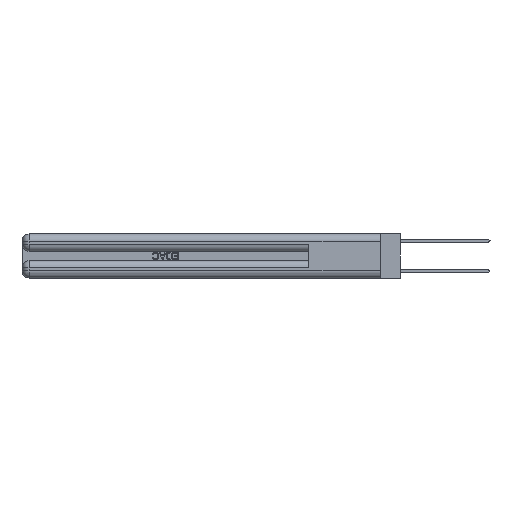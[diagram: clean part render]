
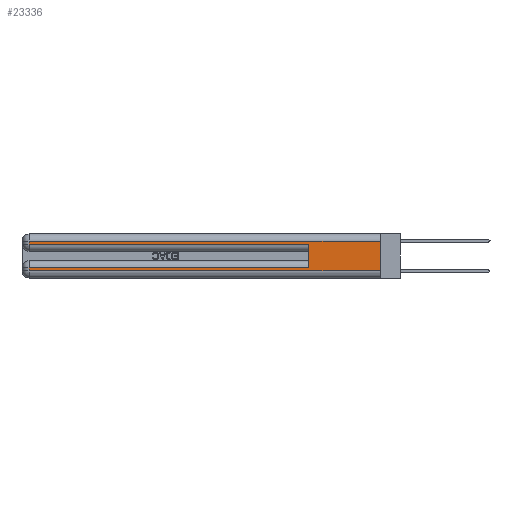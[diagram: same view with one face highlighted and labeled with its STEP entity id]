
A CAD part, left-side view. The second image highlights one B-rep face of the part: STEP entity #23336.
In plain terms, the highlighted planar face has unit normal (-1, 0, 0).
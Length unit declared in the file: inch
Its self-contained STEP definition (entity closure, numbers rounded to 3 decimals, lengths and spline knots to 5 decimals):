
#729 = EDGE_CURVE ( 'NONE', #27378, #1711, #8715, .T. ) ;
#1304 = VECTOR ( 'NONE', #10095, 39.37008 ) ;
#1372 = CARTESIAN_POINT ( 'NONE',  ( 0., 2.94, 0.285 ) ) ;
#1680 = LINE ( 'NONE', #24981, #14937 ) ;
#1711 = VERTEX_POINT ( 'NONE', #3402 ) ;
#1877 = DIRECTION ( 'NONE',  ( 0., 0., 1. ) ) ;
#3402 = CARTESIAN_POINT ( 'NONE',  ( 0., 2.94, 0.06 ) ) ;
#3909 = VECTOR ( 'NONE', #31940, 39.37008 ) ;
#4129 = EDGE_LOOP ( 'NONE', ( #23627, #28329, #7637, #20139, #12692, #15837, #10748, #32167 ) ) ;
#4683 = LINE ( 'NONE', #7664, #8990 ) ;
#4690 = LINE ( 'NONE', #29480, #3909 ) ;
#5422 = CARTESIAN_POINT ( 'NONE',  ( 0., 0., 0.37 ) ) ;
#5751 = VECTOR ( 'NONE', #10068, 39.37008 ) ;
#7191 = VERTEX_POINT ( 'NONE', #12171 ) ;
#7320 = LINE ( 'NONE', #5422, #12373 ) ;
#7637 = ORIENTED_EDGE ( 'NONE', *, *, #17892, .T. ) ;
#7664 = CARTESIAN_POINT ( 'NONE',  ( 0., 0., 0.06 ) ) ;
#7737 = EDGE_CURVE ( 'NONE', #7191, #26913, #4690, .T. ) ;
#8115 = LINE ( 'NONE', #17492, #5751 ) ;
#8715 = LINE ( 'NONE', #27445, #1304 ) ;
#8990 = VECTOR ( 'NONE', #27620, 39.37008 ) ;
#9276 = DIRECTION ( 'NONE',  ( 0., 0., -1. ) ) ;
#9380 = CARTESIAN_POINT ( 'NONE',  ( 0., 0.6, 0.145 ) ) ;
#10068 = DIRECTION ( 'NONE',  ( 0., 1., 0. ) ) ;
#10095 = DIRECTION ( 'NONE',  ( 0., 0., -1. ) ) ;
#10542 = DIRECTION ( 'NONE',  ( 0., 0., -1. ) ) ;
#10748 = ORIENTED_EDGE ( 'NONE', *, *, #729, .T. ) ;
#11470 = VECTOR ( 'NONE', #1877, 39.37008 ) ;
#12171 = CARTESIAN_POINT ( 'NONE',  ( 0., 0., 0.31 ) ) ;
#12373 = VECTOR ( 'NONE', #10542, 39.37008 ) ;
#12692 = ORIENTED_EDGE ( 'NONE', *, *, #30060, .F. ) ;
#13063 = DIRECTION ( 'NONE',  ( 1., 0., 0. ) ) ;
#14129 = FACE_OUTER_BOUND ( 'NONE', #4129, .T. ) ;
#14238 = CARTESIAN_POINT ( 'NONE',  ( 0., 2.94, 0.085 ) ) ;
#14470 = CARTESIAN_POINT ( 'NONE',  ( 0., 0., 0.06 ) ) ;
#14937 = VECTOR ( 'NONE', #27485, 39.37008 ) ;
#15837 = ORIENTED_EDGE ( 'NONE', *, *, #25826, .T. ) ;
#16109 = EDGE_CURVE ( 'NONE', #30717, #17223, #1680, .T. ) ;
#16382 = VECTOR ( 'NONE', #9276, 39.37008 ) ;
#17223 = VERTEX_POINT ( 'NONE', #26765 ) ;
#17453 = EDGE_CURVE ( 'NONE', #1711, #23746, #4683, .T. ) ;
#17492 = CARTESIAN_POINT ( 'NONE',  ( 0., 0., 0.085 ) ) ;
#17892 = EDGE_CURVE ( 'NONE', #26913, #30717, #22989, .T. ) ;
#18104 = LINE ( 'NONE', #9380, #11470 ) ;
#18151 = AXIS2_PLACEMENT_3D ( 'NONE', #28008, #13063, #30479 ) ;
#18774 = CARTESIAN_POINT ( 'NONE',  ( 0., 0.6, 0.085 ) ) ;
#19071 = CARTESIAN_POINT ( 'NONE',  ( 0., 2.94, 0.31 ) ) ;
#19201 = CARTESIAN_POINT ( 'NONE',  ( 0., 2.94, 0.37 ) ) ;
#20139 = ORIENTED_EDGE ( 'NONE', *, *, #16109, .T. ) ;
#22971 = PLANE ( 'NONE',  #18151 ) ;
#22989 = LINE ( 'NONE', #19201, #16382 ) ;
#23336 = ADVANCED_FACE ( 'NONE', ( #14129 ), #22971, .F. ) ;
#23627 = ORIENTED_EDGE ( 'NONE', *, *, #28419, .F. ) ;
#23746 = VERTEX_POINT ( 'NONE', #14470 ) ;
#24981 = CARTESIAN_POINT ( 'NONE',  ( 0., 0., 0.285 ) ) ;
#25826 = EDGE_CURVE ( 'NONE', #27901, #27378, #8115, .T. ) ;
#26765 = CARTESIAN_POINT ( 'NONE',  ( 0., 0.6, 0.285 ) ) ;
#26913 = VERTEX_POINT ( 'NONE', #19071 ) ;
#27378 = VERTEX_POINT ( 'NONE', #14238 ) ;
#27445 = CARTESIAN_POINT ( 'NONE',  ( 0., 2.94, 0.37 ) ) ;
#27485 = DIRECTION ( 'NONE',  ( 0., -1., 0. ) ) ;
#27620 = DIRECTION ( 'NONE',  ( 0., -1., 0. ) ) ;
#27901 = VERTEX_POINT ( 'NONE', #18774 ) ;
#28008 = CARTESIAN_POINT ( 'NONE',  ( 0., 0., 0.37 ) ) ;
#28329 = ORIENTED_EDGE ( 'NONE', *, *, #7737, .T. ) ;
#28419 = EDGE_CURVE ( 'NONE', #7191, #23746, #7320, .T. ) ;
#29480 = CARTESIAN_POINT ( 'NONE',  ( 0., 0., 0.31 ) ) ;
#30060 = EDGE_CURVE ( 'NONE', #27901, #17223, #18104, .T. ) ;
#30479 = DIRECTION ( 'NONE',  ( 0., 0., -1. ) ) ;
#30717 = VERTEX_POINT ( 'NONE', #1372 ) ;
#31940 = DIRECTION ( 'NONE',  ( 0., 1., 0. ) ) ;
#32167 = ORIENTED_EDGE ( 'NONE', *, *, #17453, .T. ) ;
